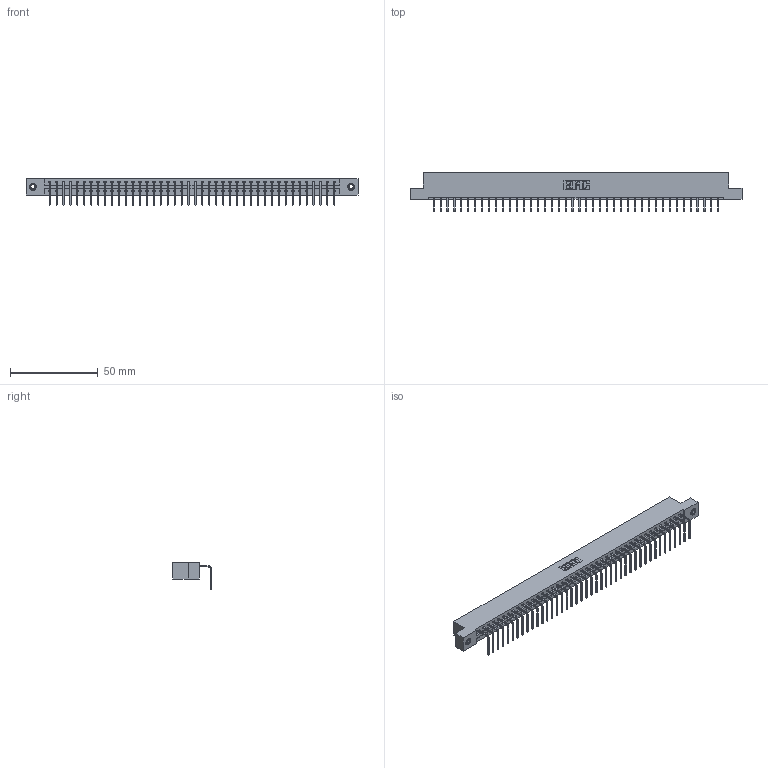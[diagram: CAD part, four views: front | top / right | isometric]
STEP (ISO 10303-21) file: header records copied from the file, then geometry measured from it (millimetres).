
FILE_DESCRIPTION (( 'STEP AP203' ), '1' );
FILE_NAME ('387-042-558-107.STEP', '2019-10-07T21:48:33', ( '' ), ( '' ), 'SwSTEP 2.0', 'SolidWorks 2016', '' );
FILE_SCHEMA (( 'CONFIG_CONTROL_DESIGN' ));
Length unit declared in the file: inch
Products named in the file (4): 337 Part_Flush Mounting Lugs - 0.156 Dia-TI; 345-250-001_345-250-005-103; 387-042-558-107; 345-292-001_558 Tail - 2
Assembly tree (45 placements, depth 2):
  387-042-558-107
    337 Part_Flush Mounting Lugs - 0.156 Dia-TI
    345-292-001_558 Tail - 2  x42
    345-250-001_345-250-005-103  x2
Bounding box: 189.43 x 22.17 x 15.37 mm (x, y, z)
Volume: 19814.8 mm3; surface area: 21376.4 mm2
Topology: 45 solids, 45 shells, 2862 faces, 8595 edges, 5666 vertices
Faces by surface type: plane 2118, cylinder 728, cone 12, torus 4
Entity records: 32490 total; most frequent: CARTESIAN_POINT 5639, ORIENTED_EDGE 5610, DIRECTION 4779, EDGE_CURVE 2805, LINE 2657, VECTOR 2657, VERTEX_POINT 1864, AXIS2_PLACEMENT_3D 1061
